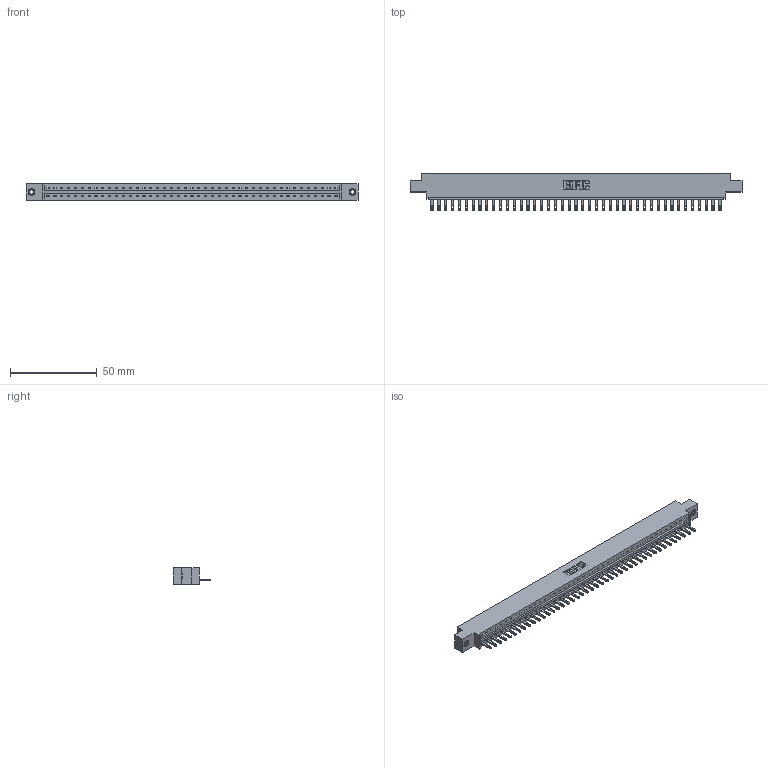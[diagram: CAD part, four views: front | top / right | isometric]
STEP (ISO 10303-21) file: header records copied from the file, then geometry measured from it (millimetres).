
FILE_DESCRIPTION (( 'STEP AP203' ), '1' );
FILE_NAME ('333-043-500-607.STEP', '2018-08-03T19:57:53', ( '' ), ( '' ), 'SwSTEP 2.0', 'SolidWorks 2016', '' );
FILE_SCHEMA (( 'CONFIG_CONTROL_DESIGN' ));
Length unit declared in the file: inch
Products named in the file (4): 333 Part_Offset - .156 Dia - TI; 345-292-001_345-293-100; 345-250-001_345-250-005-103; 333-043-500-607
Assembly tree (46 placements, depth 2):
  333-043-500-607
    333 Part_Offset - .156 Dia - TI
    345-292-001_345-293-100  x43
    345-250-001_345-250-005-103  x2
Bounding box: 191.92 x 21.85 x 9.4 mm (x, y, z)
Volume: 19106.7 mm3; surface area: 21019.7 mm2
Topology: 46 solids, 46 shells, 2500 faces, 7683 edges, 5114 vertices
Faces by surface type: plane 1654, cylinder 830, cone 12, torus 4
Entity records: 27406 total; most frequent: CARTESIAN_POINT 4710, ORIENTED_EDGE 4682, DIRECTION 4005, EDGE_CURVE 2341, LINE 2189, VECTOR 2189, VERTEX_POINT 1556, AXIS2_PLACEMENT_3D 908
